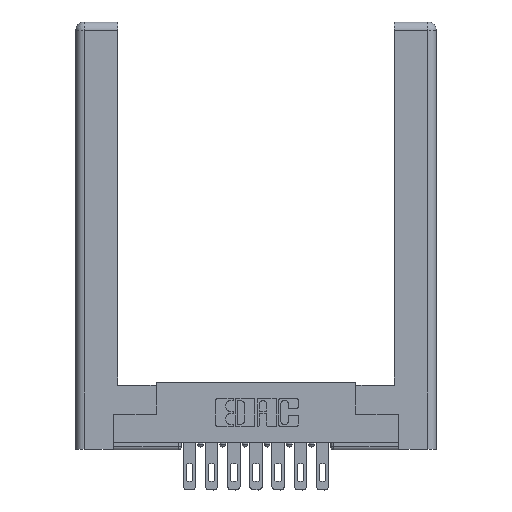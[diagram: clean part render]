
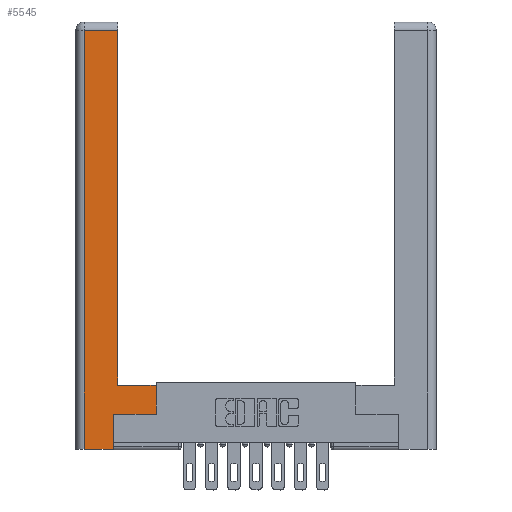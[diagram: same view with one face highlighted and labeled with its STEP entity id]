
A CAD part, top view. The second image highlights one B-rep face of the part: STEP entity #5545.
In plain terms, the highlighted planar face has unit normal (0, 0, 1).
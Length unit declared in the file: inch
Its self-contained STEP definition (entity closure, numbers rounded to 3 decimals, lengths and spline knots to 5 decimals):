
#274 = VECTOR ( 'NONE', #9817, 39.37008 ) ;
#303 = ORIENTED_EDGE ( 'NONE', *, *, #11876, .T. ) ;
#387 = CARTESIAN_POINT ( 'NONE',  ( 0.565, 0.245, 0. ) ) ;
#595 = VERTEX_POINT ( 'NONE', #7046 ) ;
#804 = EDGE_CURVE ( 'NONE', #9243, #5669, #8415, .T. ) ;
#986 = CARTESIAN_POINT ( 'NONE',  ( 0.265, 0.245, 0. ) ) ;
#1473 = CARTESIAN_POINT ( 'NONE',  ( 0.265, 0., 0. ) ) ;
#1853 = VECTOR ( 'NONE', #11977, 39.37008 ) ;
#2474 = CARTESIAN_POINT ( 'NONE',  ( 0.0615, 0., 0. ) ) ;
#2493 = LINE ( 'NONE', #2474, #5609 ) ;
#2901 = DIRECTION ( 'NONE',  ( -1., 0., 0. ) ) ;
#2943 = CARTESIAN_POINT ( 'NONE',  ( 0.565, 0.45, 0. ) ) ;
#2957 = CARTESIAN_POINT ( 'NONE',  ( 0.295, 3., 0. ) ) ;
#3452 = CARTESIAN_POINT ( 'NONE',  ( 0.295, 0.45, 0. ) ) ;
#4257 = CARTESIAN_POINT ( 'NONE',  ( 0.295, 2.94, 0. ) ) ;
#4348 = CARTESIAN_POINT ( 'NONE',  ( 0.0615, 0., 0. ) ) ;
#4702 = VERTEX_POINT ( 'NONE', #10153 ) ;
#4770 = CARTESIAN_POINT ( 'NONE',  ( 0.265, 0., 0. ) ) ;
#5090 = VERTEX_POINT ( 'NONE', #9887 ) ;
#5091 = CARTESIAN_POINT ( 'NONE',  ( 0.0615, 2.94, 0. ) ) ;
#5148 = LINE ( 'NONE', #2957, #12786 ) ;
#5545 = ADVANCED_FACE ( 'NONE', ( #5570 ), #11850, .F. ) ;
#5570 = FACE_OUTER_BOUND ( 'NONE', #5960, .T. ) ;
#5609 = VECTOR ( 'NONE', #12506, 39.37008 ) ;
#5669 = VERTEX_POINT ( 'NONE', #5091 ) ;
#5723 = VERTEX_POINT ( 'NONE', #8657 ) ;
#5865 = DIRECTION ( 'NONE',  ( 0., 1., 0. ) ) ;
#5929 = VECTOR ( 'NONE', #5865, 39.37008 ) ;
#5960 = EDGE_LOOP ( 'NONE', ( #303, #12413, #10922, #7169, #9436, #7435, #9921, #9182 ) ) ;
#6463 = DIRECTION ( 'NONE',  ( -1., 0., 0. ) ) ;
#6588 = VECTOR ( 'NONE', #6463, 39.37008 ) ;
#7046 = CARTESIAN_POINT ( 'NONE',  ( 0.265, 0.245, 0. ) ) ;
#7169 = ORIENTED_EDGE ( 'NONE', *, *, #11142, .T. ) ;
#7435 = ORIENTED_EDGE ( 'NONE', *, *, #8195, .T. ) ;
#7459 = DIRECTION ( 'NONE',  ( 1., 0., 0. ) ) ;
#7565 = DIRECTION ( 'NONE',  ( 1., 0., 0. ) ) ;
#7973 = VECTOR ( 'NONE', #7565, 39.37008 ) ;
#8195 = EDGE_CURVE ( 'NONE', #595, #5090, #9706, .T. ) ;
#8294 = LINE ( 'NONE', #3452, #6588 ) ;
#8303 = AXIS2_PLACEMENT_3D ( 'NONE', #10844, #12766, #2901 ) ;
#8415 = LINE ( 'NONE', #10484, #274 ) ;
#8591 = VERTEX_POINT ( 'NONE', #1473 ) ;
#8657 = CARTESIAN_POINT ( 'NONE',  ( 0.565, 0.45, 0. ) ) ;
#8763 = LINE ( 'NONE', #4770, #7973 ) ;
#9182 = ORIENTED_EDGE ( 'NONE', *, *, #10414, .T. ) ;
#9243 = VERTEX_POINT ( 'NONE', #4257 ) ;
#9380 = LINE ( 'NONE', #986, #5929 ) ;
#9436 = ORIENTED_EDGE ( 'NONE', *, *, #11321, .T. ) ;
#9706 = LINE ( 'NONE', #387, #11718 ) ;
#9817 = DIRECTION ( 'NONE',  ( -1., 0., 0. ) ) ;
#9887 = CARTESIAN_POINT ( 'NONE',  ( 0.565, 0.245, 0. ) ) ;
#9921 = ORIENTED_EDGE ( 'NONE', *, *, #12509, .T. ) ;
#10153 = CARTESIAN_POINT ( 'NONE',  ( 0.295, 0.45, 0. ) ) ;
#10414 = EDGE_CURVE ( 'NONE', #5723, #4702, #8294, .T. ) ;
#10484 = CARTESIAN_POINT ( 'NONE',  ( 0.0615, 2.94, 0. ) ) ;
#10844 = CARTESIAN_POINT ( 'NONE',  ( 0., 0., 0. ) ) ;
#10856 = DIRECTION ( 'NONE',  ( 0., 1., 0. ) ) ;
#10916 = LINE ( 'NONE', #2943, #1853 ) ;
#10922 = ORIENTED_EDGE ( 'NONE', *, *, #12268, .T. ) ;
#10972 = VERTEX_POINT ( 'NONE', #4348 ) ;
#11142 = EDGE_CURVE ( 'NONE', #10972, #8591, #8763, .T. ) ;
#11321 = EDGE_CURVE ( 'NONE', #8591, #595, #9380, .T. ) ;
#11718 = VECTOR ( 'NONE', #7459, 39.37008 ) ;
#11850 = PLANE ( 'NONE',  #8303 ) ;
#11876 = EDGE_CURVE ( 'NONE', #4702, #9243, #5148, .T. ) ;
#11977 = DIRECTION ( 'NONE',  ( 0., 1., 0. ) ) ;
#12268 = EDGE_CURVE ( 'NONE', #5669, #10972, #2493, .T. ) ;
#12413 = ORIENTED_EDGE ( 'NONE', *, *, #804, .T. ) ;
#12506 = DIRECTION ( 'NONE',  ( 0., -1., 0. ) ) ;
#12509 = EDGE_CURVE ( 'NONE', #5090, #5723, #10916, .T. ) ;
#12766 = DIRECTION ( 'NONE',  ( 0., 0., -1. ) ) ;
#12786 = VECTOR ( 'NONE', #10856, 39.37008 ) ;
